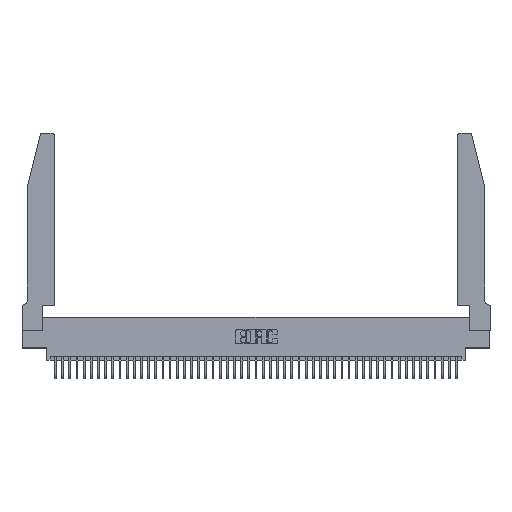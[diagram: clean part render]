
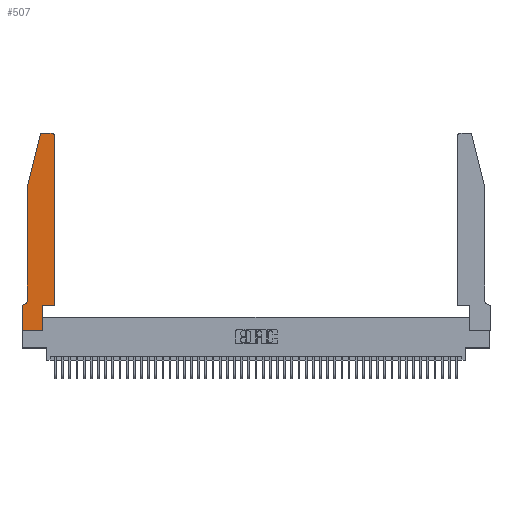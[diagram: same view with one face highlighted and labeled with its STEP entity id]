
A CAD part, top view. The second image highlights one B-rep face of the part: STEP entity #507.
In plain terms, the highlighted planar face has unit normal (0, 0, 1).
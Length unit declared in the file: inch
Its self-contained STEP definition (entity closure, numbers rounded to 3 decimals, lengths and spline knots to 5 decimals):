
#504 = EDGE_CURVE ( 'NONE', #20720, #25902, #35348, .T. ) ;
#507 = ADVANCED_FACE ( 'NONE', ( #27604 ), #38860, .T. ) ;
#1121 = CARTESIAN_POINT ( 'NONE',  ( 0.0755, 2., 0.37 ) ) ;
#1214 = VERTEX_POINT ( 'NONE', #25872 ) ;
#2047 = DIRECTION ( 'NONE',  ( 1., 0., 0. ) ) ;
#2401 = CIRCLE ( 'NONE', #12909, 0.03 ) ;
#2643 = LINE ( 'NONE', #23655, #43709 ) ;
#3377 = LINE ( 'NONE', #22230, #42620 ) ;
#3564 = EDGE_CURVE ( 'NONE', #24969, #26459, #2401, .T. ) ;
#4143 = EDGE_CURVE ( 'NONE', #29285, #1214, #14798, .T. ) ;
#4527 = CARTESIAN_POINT ( 'NONE',  ( 0., 0., 0.37 ) ) ;
#5190 = CARTESIAN_POINT ( 'NONE',  ( 0.0755, 0.42, 0.37 ) ) ;
#5849 = CARTESIAN_POINT ( 'NONE',  ( 0.4505, 0.35, 0.37 ) ) ;
#6582 = CARTESIAN_POINT ( 'NONE',  ( 0.2865, 0.35, 0.37 ) ) ;
#8226 = EDGE_CURVE ( 'NONE', #25902, #48141, #13929, .T. ) ;
#8758 = DIRECTION ( 'NONE',  ( 0., -1., 0. ) ) ;
#9445 = VECTOR ( 'NONE', #48703, 39.37008 ) ;
#9637 = AXIS2_PLACEMENT_3D ( 'NONE', #27221, #11895, #15566 ) ;
#9857 = DIRECTION ( 'NONE',  ( 0., 1., 0. ) ) ;
#11895 = DIRECTION ( 'NONE',  ( 0., 0., 1. ) ) ;
#12130 = VECTOR ( 'NONE', #8758, 39.37008 ) ;
#12576 = VECTOR ( 'NONE', #2047, 39.37008 ) ;
#12851 = DIRECTION ( 'NONE',  ( 0., 1., 0. ) ) ;
#12909 = AXIS2_PLACEMENT_3D ( 'NONE', #46226, #46059, #35067 ) ;
#12974 = ORIENTED_EDGE ( 'NONE', *, *, #44359, .T. ) ;
#13929 = CIRCLE ( 'NONE', #22577, 0.07 ) ;
#14082 = VECTOR ( 'NONE', #9857, 39.37008 ) ;
#14570 = CARTESIAN_POINT ( 'NONE',  ( 0., 0., 0.37 ) ) ;
#14798 = CIRCLE ( 'NONE', #38424, 0.03 ) ;
#15566 = DIRECTION ( 'NONE',  ( 1., 0., 0. ) ) ;
#17639 = CARTESIAN_POINT ( 'NONE',  ( 0.2865, 0.35, 0.37 ) ) ;
#17836 = VERTEX_POINT ( 'NONE', #4527 ) ;
#18181 = CARTESIAN_POINT ( 'NONE',  ( 0.284, 2.75, 0.37 ) ) ;
#18257 = DIRECTION ( 'NONE',  ( -1., 0., 0. ) ) ;
#19636 = ORIENTED_EDGE ( 'NONE', *, *, #8226, .T. ) ;
#19651 = DIRECTION ( 'NONE',  ( 1., 0., 0. ) ) ;
#20039 = VERTEX_POINT ( 'NONE', #5849 ) ;
#20720 = VERTEX_POINT ( 'NONE', #36228 ) ;
#21154 = ORIENTED_EDGE ( 'NONE', *, *, #48295, .T. ) ;
#21825 = EDGE_CURVE ( 'NONE', #26459, #20720, #2643, .T. ) ;
#21923 = LINE ( 'NONE', #14570, #9445 ) ;
#22230 = CARTESIAN_POINT ( 'NONE',  ( 0.0755, 0.35, 0.37 ) ) ;
#22274 = CARTESIAN_POINT ( 'NONE',  ( 0.2605, 2.75, 0.37 ) ) ;
#22577 = AXIS2_PLACEMENT_3D ( 'NONE', #45414, #41070, #18257 ) ;
#22673 = LINE ( 'NONE', #28639, #12576 ) ;
#23252 = ORIENTED_EDGE ( 'NONE', *, *, #49238, .T. ) ;
#23292 = ORIENTED_EDGE ( 'NONE', *, *, #46281, .T. ) ;
#23326 = DIRECTION ( 'NONE',  ( -0.239, -0.971, 0. ) ) ;
#23485 = VECTOR ( 'NONE', #19651, 39.37008 ) ;
#23618 = CARTESIAN_POINT ( 'NONE',  ( 0.4205, 2.72, 0.37 ) ) ;
#23655 = CARTESIAN_POINT ( 'NONE',  ( 0.0755, 2., 0.37 ) ) ;
#24066 = LINE ( 'NONE', #26999, #23485 ) ;
#24969 = VERTEX_POINT ( 'NONE', #18181 ) ;
#25497 = LINE ( 'NONE', #22274, #42768 ) ;
#25872 = CARTESIAN_POINT ( 'NONE',  ( 0.4205, 2.75, 0.37 ) ) ;
#25902 = VERTEX_POINT ( 'NONE', #5190 ) ;
#26459 = VERTEX_POINT ( 'NONE', #41698 ) ;
#26472 = ORIENTED_EDGE ( 'NONE', *, *, #21825, .T. ) ;
#26999 = CARTESIAN_POINT ( 'NONE',  ( 0.4505, 0.35, 0.37 ) ) ;
#27221 = CARTESIAN_POINT ( 'NONE',  ( 0., 0.35, 0.37 ) ) ;
#27604 = FACE_OUTER_BOUND ( 'NONE', #34932, .T. ) ;
#27980 = ORIENTED_EDGE ( 'NONE', *, *, #504, .T. ) ;
#28407 = ORIENTED_EDGE ( 'NONE', *, *, #41721, .T. ) ;
#28639 = CARTESIAN_POINT ( 'NONE',  ( 0., 0., 0.37 ) ) ;
#29285 = VERTEX_POINT ( 'NONE', #33060 ) ;
#29769 = ORIENTED_EDGE ( 'NONE', *, *, #43546, .T. ) ;
#32254 = CARTESIAN_POINT ( 'NONE',  ( 0.0055, 0.35, 0.37 ) ) ;
#33060 = CARTESIAN_POINT ( 'NONE',  ( 0.4505, 2.72, 0.37 ) ) ;
#33275 = ORIENTED_EDGE ( 'NONE', *, *, #4143, .T. ) ;
#34917 = LINE ( 'NONE', #41972, #42631 ) ;
#34932 = EDGE_LOOP ( 'NONE', ( #28407, #45118, #26472, #27980, #19636, #29769, #23252, #21154, #44371, #23292, #12974, #33275 ) ) ;
#35067 = DIRECTION ( 'NONE',  ( 1., 0., 0. ) ) ;
#35114 = DIRECTION ( 'NONE',  ( 1., 0., 0. ) ) ;
#35341 = CARTESIAN_POINT ( 'NONE',  ( 0.2865, 0., 0.37 ) ) ;
#35348 = LINE ( 'NONE', #1121, #12130 ) ;
#36057 = VERTEX_POINT ( 'NONE', #6582 ) ;
#36228 = CARTESIAN_POINT ( 'NONE',  ( 0.0755, 2., 0.37 ) ) ;
#37224 = DIRECTION ( 'NONE',  ( -1., 0., 0. ) ) ;
#38424 = AXIS2_PLACEMENT_3D ( 'NONE', #23618, #38441, #35114 ) ;
#38441 = DIRECTION ( 'NONE',  ( 0., 0., 1. ) ) ;
#38596 = VERTEX_POINT ( 'NONE', #35341 ) ;
#38860 = PLANE ( 'NONE',  #9637 ) ;
#40290 = VERTEX_POINT ( 'NONE', #44391 ) ;
#41070 = DIRECTION ( 'NONE',  ( 0., 0., -1. ) ) ;
#41414 = DIRECTION ( 'NONE',  ( -1., 0., 0. ) ) ;
#41698 = CARTESIAN_POINT ( 'NONE',  ( 0.25487, 2.72718, 0.37 ) ) ;
#41721 = EDGE_CURVE ( 'NONE', #1214, #24969, #25497, .T. ) ;
#41972 = CARTESIAN_POINT ( 'NONE',  ( 0.4505, 0.35, 0.37 ) ) ;
#42620 = VECTOR ( 'NONE', #37224, 39.37008 ) ;
#42631 = VECTOR ( 'NONE', #12851, 39.37008 ) ;
#42768 = VECTOR ( 'NONE', #41414, 39.37008 ) ;
#43546 = EDGE_CURVE ( 'NONE', #48141, #40290, #3377, .T. ) ;
#43709 = VECTOR ( 'NONE', #23326, 39.37008 ) ;
#44359 = EDGE_CURVE ( 'NONE', #20039, #29285, #34917, .T. ) ;
#44371 = ORIENTED_EDGE ( 'NONE', *, *, #44573, .T. ) ;
#44391 = CARTESIAN_POINT ( 'NONE',  ( 0., 0.35, 0.37 ) ) ;
#44451 = LINE ( 'NONE', #17639, #14082 ) ;
#44573 = EDGE_CURVE ( 'NONE', #38596, #36057, #44451, .T. ) ;
#45118 = ORIENTED_EDGE ( 'NONE', *, *, #3564, .T. ) ;
#45414 = CARTESIAN_POINT ( 'NONE',  ( 0.0055, 0.42, 0.37 ) ) ;
#46059 = DIRECTION ( 'NONE',  ( 0., 0., 1. ) ) ;
#46226 = CARTESIAN_POINT ( 'NONE',  ( 0.284, 2.72, 0.37 ) ) ;
#46281 = EDGE_CURVE ( 'NONE', #36057, #20039, #24066, .T. ) ;
#48141 = VERTEX_POINT ( 'NONE', #32254 ) ;
#48295 = EDGE_CURVE ( 'NONE', #17836, #38596, #22673, .T. ) ;
#48703 = DIRECTION ( 'NONE',  ( 0., -1., 0. ) ) ;
#49238 = EDGE_CURVE ( 'NONE', #40290, #17836, #21923, .T. ) ;
